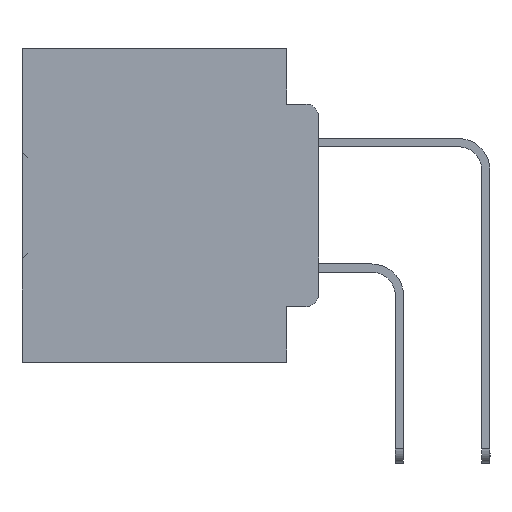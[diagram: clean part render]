
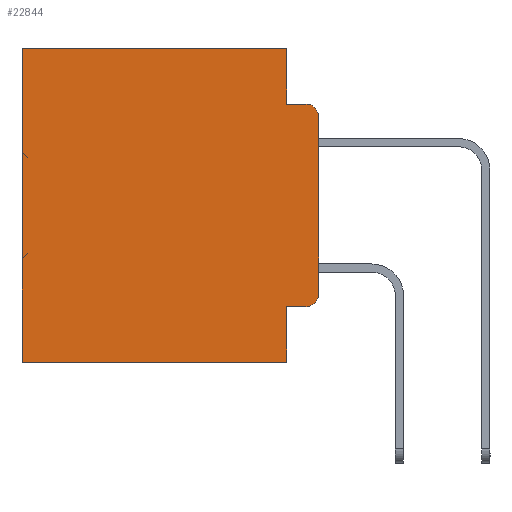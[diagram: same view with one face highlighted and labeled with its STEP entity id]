
A CAD part, left-side view. The second image highlights one B-rep face of the part: STEP entity #22844.
In plain terms, the highlighted planar face has unit normal (-1, 0, 0).
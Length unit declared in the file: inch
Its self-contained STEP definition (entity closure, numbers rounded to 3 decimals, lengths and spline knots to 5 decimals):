
#56 = EDGE_CURVE ( 'NONE', #16248, #31118, #38046, .T. ) ;
#565 = CARTESIAN_POINT ( 'NONE',  ( 0.298, 0.02, -0.1085 ) ) ;
#624 = ORIENTED_EDGE ( 'NONE', *, *, #5692, .F. ) ;
#677 = CARTESIAN_POINT ( 'NONE',  ( 0.298, 0.051, 0. ) ) ;
#797 = EDGE_CURVE ( 'NONE', #24685, #38809, #38911, .T. ) ;
#2085 = VECTOR ( 'NONE', #39505, 39.37008 ) ;
#2211 = DIRECTION ( 'NONE',  ( 1., 0., 0. ) ) ;
#2677 = VECTOR ( 'NONE', #17021, 39.37008 ) ;
#2746 = CARTESIAN_POINT ( 'NONE',  ( 0.298, 0., -0.3915 ) ) ;
#2994 = VERTEX_POINT ( 'NONE', #26237 ) ;
#3038 = VECTOR ( 'NONE', #12774, 39.37008 ) ;
#3066 = AXIS2_PLACEMENT_3D ( 'NONE', #24600, #36758, #21551 ) ;
#5692 = EDGE_CURVE ( 'NONE', #32068, #38104, #20478, .T. ) ;
#6128 = VECTOR ( 'NONE', #19695, 39.37008 ) ;
#6352 = CARTESIAN_POINT ( 'NONE',  ( 0.298, 0., -0.1085 ) ) ;
#6654 = CARTESIAN_POINT ( 'NONE',  ( 0.298, 0., 0. ) ) ;
#6656 = DIRECTION ( 'NONE',  ( 0., 0., -1. ) ) ;
#7118 = EDGE_CURVE ( 'NONE', #21956, #31118, #11957, .T. ) ;
#7372 = VERTEX_POINT ( 'NONE', #33947 ) ;
#7875 = LINE ( 'NONE', #17431, #2677 ) ;
#9507 = DIRECTION ( 'NONE',  ( -1., 0., 0. ) ) ;
#10588 = EDGE_CURVE ( 'NONE', #17780, #38809, #28187, .T. ) ;
#11227 = EDGE_CURVE ( 'NONE', #7372, #32068, #28540, .T. ) ;
#11957 = LINE ( 'NONE', #6654, #35835 ) ;
#12658 = LINE ( 'NONE', #677, #35935 ) ;
#12774 = DIRECTION ( 'NONE',  ( 0., 0., -1. ) ) ;
#13573 = ORIENTED_EDGE ( 'NONE', *, *, #797, .F. ) ;
#14599 = DIRECTION ( 'NONE',  ( 0., 0., -1. ) ) ;
#16248 = VERTEX_POINT ( 'NONE', #16770 ) ;
#16770 = CARTESIAN_POINT ( 'NONE',  ( 0.298, 0.02, -0.4115 ) ) ;
#17021 = DIRECTION ( 'NONE',  ( 0., -1., 0. ) ) ;
#17260 = LINE ( 'NONE', #32438, #6128 ) ;
#17431 = CARTESIAN_POINT ( 'NONE',  ( 0.298, 0.051, -0.4115 ) ) ;
#17772 = EDGE_CURVE ( 'NONE', #2994, #24685, #12658, .T. ) ;
#17780 = VERTEX_POINT ( 'NONE', #25447 ) ;
#19695 = DIRECTION ( 'NONE',  ( 0., 1., 0. ) ) ;
#20478 = LINE ( 'NONE', #29790, #2085 ) ;
#21551 = DIRECTION ( 'NONE',  ( 0., 0., -1. ) ) ;
#21956 = VERTEX_POINT ( 'NONE', #6352 ) ;
#22844 = ADVANCED_FACE ( 'NONE', ( #33220 ), #36073, .F. ) ;
#22917 = CARTESIAN_POINT ( 'NONE',  ( 0.298, 0., -0.5 ) ) ;
#23576 = EDGE_LOOP ( 'NONE', ( #26223, #28343, #624, #33667, #32436, #36091, #13573, #37070, #35917, #36474 ) ) ;
#24294 = EDGE_CURVE ( 'NONE', #21956, #38104, #32978, .T. ) ;
#24588 = AXIS2_PLACEMENT_3D ( 'NONE', #33025, #2211, #14599 ) ;
#24600 = CARTESIAN_POINT ( 'NONE',  ( 0.298, 0.02, -0.3915 ) ) ;
#24685 = VERTEX_POINT ( 'NONE', #39004 ) ;
#25447 = CARTESIAN_POINT ( 'NONE',  ( 0.298, 0.473, 0. ) ) ;
#26223 = ORIENTED_EDGE ( 'NONE', *, *, #7118, .F. ) ;
#26237 = CARTESIAN_POINT ( 'NONE',  ( 0.298, 0.051, -0.4115 ) ) ;
#27179 = CARTESIAN_POINT ( 'NONE',  ( 0.298, 0.02, -0.0885 ) ) ;
#28187 = LINE ( 'NONE', #39949, #3038 ) ;
#28343 = ORIENTED_EDGE ( 'NONE', *, *, #24294, .T. ) ;
#28540 = LINE ( 'NONE', #38074, #30194 ) ;
#29113 = EDGE_CURVE ( 'NONE', #2994, #16248, #7875, .T. ) ;
#29512 = CARTESIAN_POINT ( 'NONE',  ( 0.298, 0.473, -0.5 ) ) ;
#29790 = CARTESIAN_POINT ( 'NONE',  ( 0.298, 0.051, -0.0885 ) ) ;
#30194 = VECTOR ( 'NONE', #32374, 39.37008 ) ;
#30994 = DIRECTION ( 'NONE',  ( 0., 0., -1. ) ) ;
#31118 = VERTEX_POINT ( 'NONE', #2746 ) ;
#32068 = VERTEX_POINT ( 'NONE', #33273 ) ;
#32374 = DIRECTION ( 'NONE',  ( 0., 0., -1. ) ) ;
#32436 = ORIENTED_EDGE ( 'NONE', *, *, #33538, .T. ) ;
#32438 = CARTESIAN_POINT ( 'NONE',  ( 0.298, 0., 0. ) ) ;
#32978 = CIRCLE ( 'NONE', #38164, 0.02 ) ;
#33025 = CARTESIAN_POINT ( 'NONE',  ( 0.298, 0., 0. ) ) ;
#33220 = FACE_OUTER_BOUND ( 'NONE', #23576, .T. ) ;
#33273 = CARTESIAN_POINT ( 'NONE',  ( 0.298, 0.051, -0.0885 ) ) ;
#33538 = EDGE_CURVE ( 'NONE', #7372, #17780, #17260, .T. ) ;
#33667 = ORIENTED_EDGE ( 'NONE', *, *, #11227, .F. ) ;
#33947 = CARTESIAN_POINT ( 'NONE',  ( 0.298, 0.051, 0. ) ) ;
#34541 = DIRECTION ( 'NONE',  ( 0., 0., -1. ) ) ;
#35102 = VECTOR ( 'NONE', #39113, 39.37008 ) ;
#35835 = VECTOR ( 'NONE', #30994, 39.37008 ) ;
#35917 = ORIENTED_EDGE ( 'NONE', *, *, #29113, .T. ) ;
#35935 = VECTOR ( 'NONE', #34541, 39.37008 ) ;
#36073 = PLANE ( 'NONE',  #24588 ) ;
#36091 = ORIENTED_EDGE ( 'NONE', *, *, #10588, .T. ) ;
#36474 = ORIENTED_EDGE ( 'NONE', *, *, #56, .T. ) ;
#36758 = DIRECTION ( 'NONE',  ( -1., 0., 0. ) ) ;
#37070 = ORIENTED_EDGE ( 'NONE', *, *, #17772, .F. ) ;
#38046 = CIRCLE ( 'NONE', #3066, 0.02 ) ;
#38074 = CARTESIAN_POINT ( 'NONE',  ( 0.298, 0.051, 0. ) ) ;
#38104 = VERTEX_POINT ( 'NONE', #27179 ) ;
#38164 = AXIS2_PLACEMENT_3D ( 'NONE', #565, #9507, #6656 ) ;
#38809 = VERTEX_POINT ( 'NONE', #29512 ) ;
#38911 = LINE ( 'NONE', #22917, #35102 ) ;
#39004 = CARTESIAN_POINT ( 'NONE',  ( 0.298, 0.051, -0.5 ) ) ;
#39113 = DIRECTION ( 'NONE',  ( 0., 1., 0. ) ) ;
#39505 = DIRECTION ( 'NONE',  ( 0., -1., 0. ) ) ;
#39949 = CARTESIAN_POINT ( 'NONE',  ( 0.298, 0.473, 0. ) ) ;
